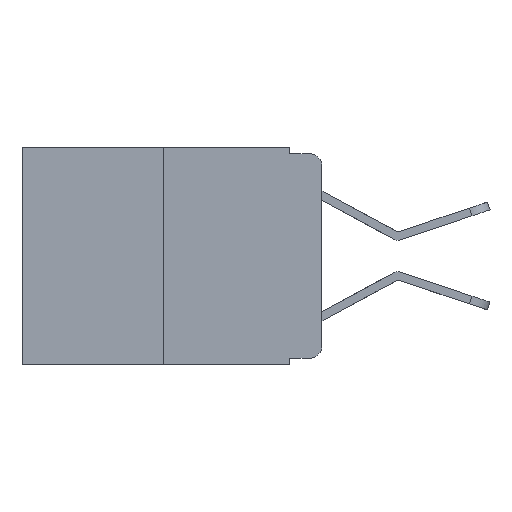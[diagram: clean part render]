
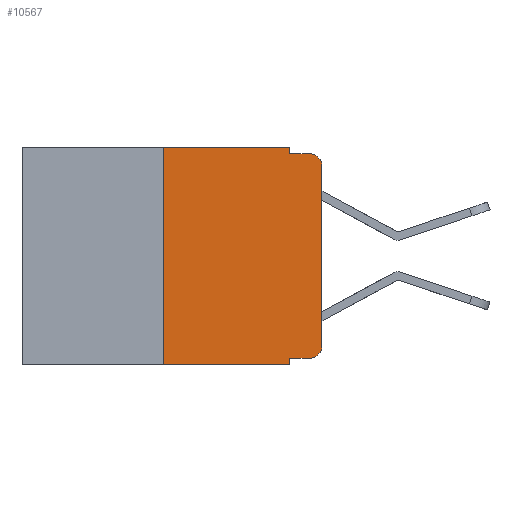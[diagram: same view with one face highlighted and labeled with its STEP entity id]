
A CAD part, left-side view. The second image highlights one B-rep face of the part: STEP entity #10567.
In plain terms, the highlighted planar face has unit normal (-1, 0, 0).
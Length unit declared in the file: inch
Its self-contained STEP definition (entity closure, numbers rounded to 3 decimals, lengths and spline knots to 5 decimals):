
#205 = CARTESIAN_POINT ( 'NONE',  ( 0., 0.473, -0.343 ) ) ;
#370 = DIRECTION ( 'NONE',  ( 0., -1., 0. ) ) ;
#994 = ORIENTED_EDGE ( 'NONE', *, *, #12062, .F. ) ;
#1043 = VECTOR ( 'NONE', #14627, 39.37008 ) ;
#1262 = DIRECTION ( 'NONE',  ( 0., 0., 1. ) ) ;
#1928 = CARTESIAN_POINT ( 'NONE',  ( 0., 0.051, -0.01 ) ) ;
#3002 = CARTESIAN_POINT ( 'NONE',  ( 0., 0.25, 0. ) ) ;
#3791 = EDGE_CURVE ( 'NONE', #19722, #23715, #18697, .T. ) ;
#3793 = ORIENTED_EDGE ( 'NONE', *, *, #15707, .T. ) ;
#4057 = DIRECTION ( 'NONE',  ( 0., 0., -1. ) ) ;
#4682 = ORIENTED_EDGE ( 'NONE', *, *, #22390, .F. ) ;
#4704 = DIRECTION ( 'NONE',  ( 0., 0., -1. ) ) ;
#4783 = CARTESIAN_POINT ( 'NONE',  ( 0., 0.02, -0.313 ) ) ;
#4964 = LINE ( 'NONE', #17871, #14145 ) ;
#5157 = ORIENTED_EDGE ( 'NONE', *, *, #5333, .F. ) ;
#5333 = EDGE_CURVE ( 'NONE', #19722, #21611, #21206, .T. ) ;
#5437 = VECTOR ( 'NONE', #21659, 39.37008 ) ;
#5797 = CIRCLE ( 'NONE', #10372, 0.02 ) ;
#5974 = VECTOR ( 'NONE', #8216, 39.37008 ) ;
#6049 = VERTEX_POINT ( 'NONE', #8900 ) ;
#6067 = CARTESIAN_POINT ( 'NONE',  ( 0., 0.25, 0. ) ) ;
#6117 = CARTESIAN_POINT ( 'NONE',  ( 0., 0.051, -0.01 ) ) ;
#6881 = DIRECTION ( 'NONE',  ( 0., 0., -1. ) ) ;
#7268 = CARTESIAN_POINT ( 'NONE',  ( 0., 0.051, -0.333 ) ) ;
#7384 = VECTOR ( 'NONE', #13755, 39.37008 ) ;
#7765 = LINE ( 'NONE', #16023, #5437 ) ;
#7854 = DIRECTION ( 'NONE',  ( 0., 0., -1. ) ) ;
#8216 = DIRECTION ( 'NONE',  ( 0., -1., 0. ) ) ;
#8532 = VECTOR ( 'NONE', #4057, 39.37008 ) ;
#8588 = VERTEX_POINT ( 'NONE', #8703 ) ;
#8703 = CARTESIAN_POINT ( 'NONE',  ( 0., 0., -0.313 ) ) ;
#8900 = CARTESIAN_POINT ( 'NONE',  ( 0., 0.02, -0.333 ) ) ;
#9482 = VECTOR ( 'NONE', #1262, 39.37008 ) ;
#10016 = VERTEX_POINT ( 'NONE', #23748 ) ;
#10237 = VERTEX_POINT ( 'NONE', #15152 ) ;
#10372 = AXIS2_PLACEMENT_3D ( 'NONE', #22451, #13386, #7854 ) ;
#10567 = ADVANCED_FACE ( 'NONE', ( #20805 ), #16667, .F. ) ;
#11045 = CARTESIAN_POINT ( 'NONE',  ( 0., 0.473, 0. ) ) ;
#11123 = DIRECTION ( 'NONE',  ( 0., 0., -1. ) ) ;
#11290 = DIRECTION ( 'NONE',  ( 1., 0., 0. ) ) ;
#11741 = LINE ( 'NONE', #6117, #5974 ) ;
#11862 = EDGE_CURVE ( 'NONE', #21611, #12276, #7765, .T. ) ;
#11919 = CARTESIAN_POINT ( 'NONE',  ( 0., 0., 0. ) ) ;
#12062 = EDGE_CURVE ( 'NONE', #10016, #23715, #13965, .T. ) ;
#12196 = CARTESIAN_POINT ( 'NONE',  ( 0., 0.051, -0.343 ) ) ;
#12276 = VERTEX_POINT ( 'NONE', #19377 ) ;
#12302 = VERTEX_POINT ( 'NONE', #1928 ) ;
#13045 = EDGE_CURVE ( 'NONE', #10016, #6049, #13664, .T. ) ;
#13109 = LINE ( 'NONE', #11919, #7384 ) ;
#13386 = DIRECTION ( 'NONE',  ( -1., 0., 0. ) ) ;
#13664 = LINE ( 'NONE', #7268, #1043 ) ;
#13755 = DIRECTION ( 'NONE',  ( 0., 0., 1. ) ) ;
#13889 = EDGE_LOOP ( 'NONE', ( #20923, #20417, #15689, #4682, #22933, #5157, #21306, #994, #20843, #3793 ) ) ;
#13965 = LINE ( 'NONE', #15051, #8532 ) ;
#14145 = VECTOR ( 'NONE', #6881, 39.37008 ) ;
#14627 = DIRECTION ( 'NONE',  ( 0., -1., 0. ) ) ;
#15051 = CARTESIAN_POINT ( 'NONE',  ( 0., 0.051, 0. ) ) ;
#15152 = CARTESIAN_POINT ( 'NONE',  ( 0., 0., -0.03 ) ) ;
#15262 = AXIS2_PLACEMENT_3D ( 'NONE', #4783, #17866, #4704 ) ;
#15445 = EDGE_CURVE ( 'NONE', #10237, #18926, #5797, .T. ) ;
#15689 = ORIENTED_EDGE ( 'NONE', *, *, #17001, .F. ) ;
#15707 = EDGE_CURVE ( 'NONE', #6049, #8588, #18104, .T. ) ;
#16023 = CARTESIAN_POINT ( 'NONE',  ( 0., 0.473, 0. ) ) ;
#16667 = PLANE ( 'NONE',  #22581 ) ;
#17001 = EDGE_CURVE ( 'NONE', #12302, #18926, #11741, .T. ) ;
#17019 = CARTESIAN_POINT ( 'NONE',  ( 0., 0.02, -0.01 ) ) ;
#17825 = VECTOR ( 'NONE', #370, 39.37008 ) ;
#17866 = DIRECTION ( 'NONE',  ( -1., 0., 0. ) ) ;
#17871 = CARTESIAN_POINT ( 'NONE',  ( 0., 0.051, 0. ) ) ;
#18104 = CIRCLE ( 'NONE', #15262, 0.02 ) ;
#18697 = LINE ( 'NONE', #205, #17825 ) ;
#18926 = VERTEX_POINT ( 'NONE', #17019 ) ;
#19377 = CARTESIAN_POINT ( 'NONE',  ( 0., 0.051, 0. ) ) ;
#19722 = VERTEX_POINT ( 'NONE', #22118 ) ;
#19944 = EDGE_CURVE ( 'NONE', #8588, #10237, #13109, .T. ) ;
#20417 = ORIENTED_EDGE ( 'NONE', *, *, #15445, .T. ) ;
#20805 = FACE_OUTER_BOUND ( 'NONE', #13889, .T. ) ;
#20843 = ORIENTED_EDGE ( 'NONE', *, *, #13045, .T. ) ;
#20923 = ORIENTED_EDGE ( 'NONE', *, *, #19944, .T. ) ;
#21206 = LINE ( 'NONE', #3002, #9482 ) ;
#21306 = ORIENTED_EDGE ( 'NONE', *, *, #3791, .T. ) ;
#21611 = VERTEX_POINT ( 'NONE', #6067 ) ;
#21659 = DIRECTION ( 'NONE',  ( 0., -1., 0. ) ) ;
#22118 = CARTESIAN_POINT ( 'NONE',  ( 0., 0.25, -0.343 ) ) ;
#22390 = EDGE_CURVE ( 'NONE', #12276, #12302, #4964, .T. ) ;
#22451 = CARTESIAN_POINT ( 'NONE',  ( 0., 0.02, -0.03 ) ) ;
#22581 = AXIS2_PLACEMENT_3D ( 'NONE', #11045, #11290, #11123 ) ;
#22933 = ORIENTED_EDGE ( 'NONE', *, *, #11862, .F. ) ;
#23715 = VERTEX_POINT ( 'NONE', #12196 ) ;
#23748 = CARTESIAN_POINT ( 'NONE',  ( 0., 0.051, -0.333 ) ) ;
